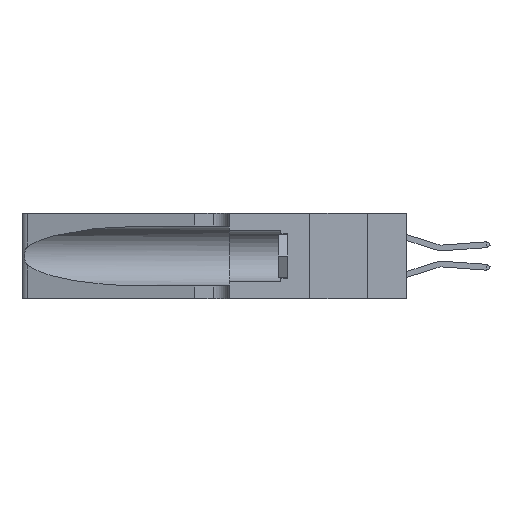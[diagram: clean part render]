
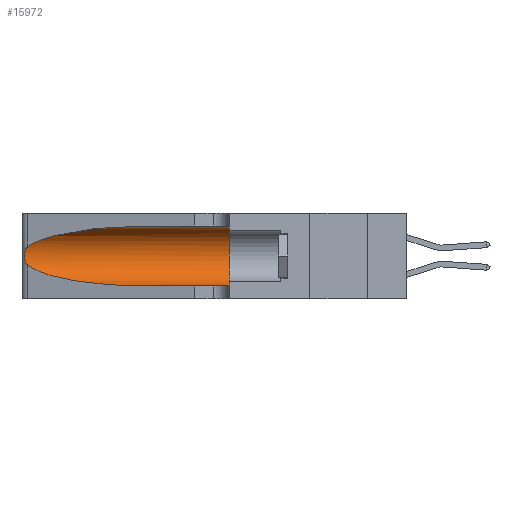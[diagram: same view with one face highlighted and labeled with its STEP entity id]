
A CAD part, left-side view. The second image highlights one B-rep face of the part: STEP entity #15972.
In plain terms, the highlighted cylindrical face has radius 3.308 mm (diameter 6.617 mm), a partial arc.
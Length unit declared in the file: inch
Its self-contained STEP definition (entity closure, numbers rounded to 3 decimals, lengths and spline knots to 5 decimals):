
#575 = VECTOR ( 'NONE', #1533, 39.37008 ) ;
#1533 = DIRECTION ( 'NONE',  ( 0., -1., 0. ) ) ;
#1563 = VERTEX_POINT ( 'NONE', #14799 ) ;
#1820 = VECTOR ( 'NONE', #7033, 39.37008 ) ;
#1912 = VERTEX_POINT ( 'NONE', #8323 ) ;
#2487 = CARTESIAN_POINT ( 'NONE',  ( 0.18966, 0.96281, 0.31525 ) ) ;
#2761 = DIRECTION ( 'NONE',  ( 0., 0., -1. ) ) ;
#2769 = CARTESIAN_POINT ( 'NONE',  ( 0.26017, 1.23833, 0.17102 ) ) ;
#4419 = VERTEX_POINT ( 'NONE', #18753 ) ;
#4492 = EDGE_CURVE ( 'NONE', #26129, #1563, #12646, .T. ) ;
#5184 = CARTESIAN_POINT ( 'NONE',  ( 0.25487, 1.22718, 0.14631 ) ) ;
#5277 = CARTESIAN_POINT ( 'NONE',  ( 0.25789, 1.23486, 0.15765 ) ) ;
#5351 = CARTESIAN_POINT ( 'NONE',  ( 0.25787, 1.23484, 0.2124 ) ) ;
#6501 = CARTESIAN_POINT ( 'NONE',  ( 0.25487, 1.22718, 0.14631 ) ) ;
#7033 = DIRECTION ( 'NONE',  ( 0., -1., 0. ) ) ;
#7063 = AXIS2_PLACEMENT_3D ( 'NONE', #14293, #18956, #2761 ) ;
#7786 = CARTESIAN_POINT ( 'NONE',  ( 0.25487, 1.22718, 0.22369 ) ) ;
#8323 = CARTESIAN_POINT ( 'NONE',  ( 0.1305, 0.72297, 0.05475 ) ) ;
#8721 = EDGE_CURVE ( 'NONE', #16570, #1912, #15541, .T. ) ;
#9268 = DIRECTION ( 'NONE',  ( 0., 0., 1. ) ) ;
#9333 = B_SPLINE_CURVE_WITH_KNOTS ( 'NONE', 3,
 ( #7786, #14269, #19291, #5351, #9898, #12342, #17217, #9689, #2769, #17454, #5277, #13286, #21269, #5184 ),
 .UNSPECIFIED., .F., .F.,
 ( 4, 2, 2, 2, 2, 2, 4 ),
 ( 0., 0.00027, 0.00053, 0.00107, 0.0016, 0.00187, 0.00214 ),
 .UNSPECIFIED. ) ;
#9348 = CARTESIAN_POINT ( 'NONE',  ( 0.1305, 1.61858, 0.31525 ) ) ;
#9666 = ORIENTED_EDGE ( 'NONE', *, *, #4492, .F. ) ;
#9689 = CARTESIAN_POINT ( 'NONE',  ( 0.26075, 1.23896, 0.178 ) ) ;
#9898 = CARTESIAN_POINT ( 'NONE',  ( 0.25854, 1.2359, 0.20912 ) ) ;
#10240 = CIRCLE ( 'NONE', #10711, 0.13025 ) ;
#10711 = AXIS2_PLACEMENT_3D ( 'NONE', #11029, #23433, #9268 ) ;
#10775 = CARTESIAN_POINT ( 'NONE',  ( 0.25487, 1.22718, 0.22369 ) ) ;
#11029 = CARTESIAN_POINT ( 'NONE',  ( 0.1305, 0.35, 0.185 ) ) ;
#12269 = CARTESIAN_POINT ( 'NONE',  ( 0.1305, 0.72297, 0.31525 ) ) ;
#12342 = CARTESIAN_POINT ( 'NONE',  ( 0.26018, 1.23835, 0.19895 ) ) ;
#12646 = LINE ( 'NONE', #9348, #1820 ) ;
#12816 = CARTESIAN_POINT ( 'NONE',  ( 0.25487, 1.22718, 0.22369 ) ) ;
#12944 = EDGE_CURVE ( 'NONE', #1912, #4419, #15224, .T. ) ;
#13286 = CARTESIAN_POINT ( 'NONE',  ( 0.25639, 1.23186, 0.15144 ) ) ;
#13377 = CYLINDRICAL_SURFACE ( 'NONE', #7063, 0.13025 ) ;
#14269 = CARTESIAN_POINT ( 'NONE',  ( 0.25555, 1.22994, 0.2215 ) ) ;
#14293 = CARTESIAN_POINT ( 'NONE',  ( 0.1305, 1.61858, 0.185 ) ) ;
#14332 = FACE_OUTER_BOUND ( 'NONE', #21336, .T. ) ;
#14605 = CARTESIAN_POINT ( 'NONE',  ( 0.2373, 1.15595, 0.08982 ) ) ;
#14690 = CARTESIAN_POINT ( 'NONE',  ( 0.1305, 0.72297, 0.05475 ) ) ;
#14756 = ORIENTED_EDGE ( 'NONE', *, *, #21457, .F. ) ;
#14799 = CARTESIAN_POINT ( 'NONE',  ( 0.1305, 0.35, 0.31525 ) ) ;
#15057 = ORIENTED_EDGE ( 'NONE', *, *, #8721, .T. ) ;
#15148 = CARTESIAN_POINT ( 'NONE',  ( 0.2373, 1.15595, 0.28018 ) ) ;
#15224 = LINE ( 'NONE', #25880, #575 ) ;
#15287 = ORIENTED_EDGE ( 'NONE', *, *, #18014, .T. ) ;
#15541 =( BOUNDED_CURVE ( )  B_SPLINE_CURVE ( 3, ( #6501, #14605, #24919, #14690 ),
 .UNSPECIFIED., .F., .F. ) 
 B_SPLINE_CURVE_WITH_KNOTS ( ( 4, 4 ),
 ( 3.44316, 4.71239 ),
 .UNSPECIFIED. ) 
 CURVE ( )  GEOMETRIC_REPRESENTATION_ITEM ( )  RATIONAL_B_SPLINE_CURVE ( ( 1., 0.87, 0.87, 1. ) ) 
 REPRESENTATION_ITEM ( '' )  );
#15972 = ADVANCED_FACE ( 'NONE', ( #14332 ), #13377, .F. ) ;
#16312 = VERTEX_POINT ( 'NONE', #10775 ) ;
#16570 = VERTEX_POINT ( 'NONE', #17000 ) ;
#17000 = CARTESIAN_POINT ( 'NONE',  ( 0.25487, 1.22718, 0.14631 ) ) ;
#17217 = CARTESIAN_POINT ( 'NONE',  ( 0.26075, 1.23896, 0.19203 ) ) ;
#17454 = CARTESIAN_POINT ( 'NONE',  ( 0.25856, 1.23593, 0.16098 ) ) ;
#17975 = ORIENTED_EDGE ( 'NONE', *, *, #12944, .T. ) ;
#18014 = EDGE_CURVE ( 'NONE', #26129, #16312, #24119, .T. ) ;
#18610 = CARTESIAN_POINT ( 'NONE',  ( 0.1305, 0.72297, 0.31525 ) ) ;
#18753 = CARTESIAN_POINT ( 'NONE',  ( 0.1305, 0.35, 0.05475 ) ) ;
#18956 = DIRECTION ( 'NONE',  ( 0., -1., 0. ) ) ;
#19243 = ORIENTED_EDGE ( 'NONE', *, *, #21207, .T. ) ;
#19291 = CARTESIAN_POINT ( 'NONE',  ( 0.25639, 1.23184, 0.21858 ) ) ;
#21207 = EDGE_CURVE ( 'NONE', #16312, #16570, #9333, .T. ) ;
#21269 = CARTESIAN_POINT ( 'NONE',  ( 0.25555, 1.22993, 0.14849 ) ) ;
#21336 = EDGE_LOOP ( 'NONE', ( #15287, #19243, #15057, #17975, #14756, #9666 ) ) ;
#21457 = EDGE_CURVE ( 'NONE', #1563, #4419, #10240, .T. ) ;
#23433 = DIRECTION ( 'NONE',  ( 0., 1., 0. ) ) ;
#24119 =( BOUNDED_CURVE ( )  B_SPLINE_CURVE ( 3, ( #18610, #2487, #15148, #12816 ),
 .UNSPECIFIED., .F., .T. ) 
 B_SPLINE_CURVE_WITH_KNOTS ( ( 4, 4 ),
 ( 1.5708, 2.84003 ),
 .UNSPECIFIED. ) 
 CURVE ( )  GEOMETRIC_REPRESENTATION_ITEM ( )  RATIONAL_B_SPLINE_CURVE ( ( 1., 0.87, 0.87, 1. ) ) 
 REPRESENTATION_ITEM ( '' )  );
#24919 = CARTESIAN_POINT ( 'NONE',  ( 0.18966, 0.96281, 0.05475 ) ) ;
#25880 = CARTESIAN_POINT ( 'NONE',  ( 0.1305, 1.61858, 0.05475 ) ) ;
#26129 = VERTEX_POINT ( 'NONE', #12269 ) ;
